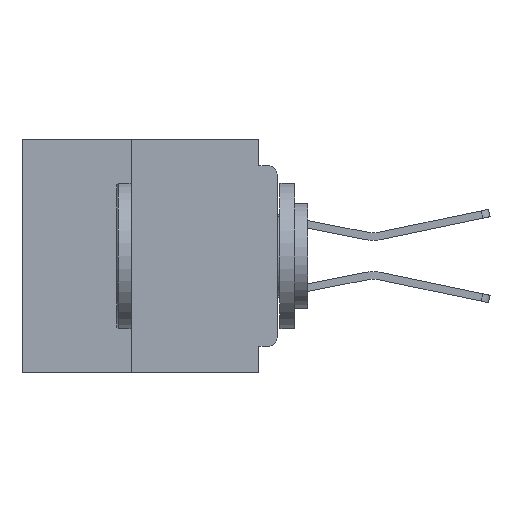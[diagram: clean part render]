
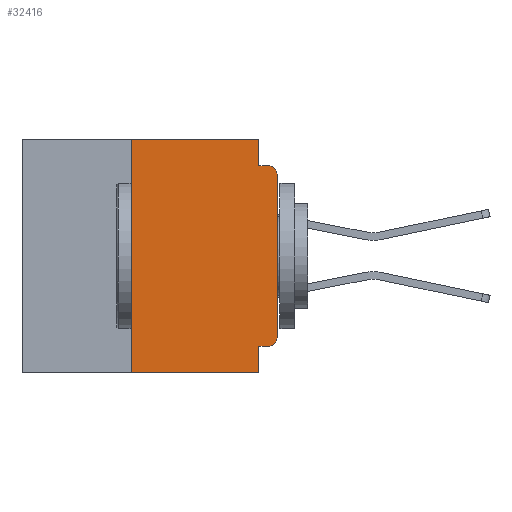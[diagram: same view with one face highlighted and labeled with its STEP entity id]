
A CAD part, left-side view. The second image highlights one B-rep face of the part: STEP entity #32416.
In plain terms, the highlighted planar face has unit normal (-1, 0, 0).
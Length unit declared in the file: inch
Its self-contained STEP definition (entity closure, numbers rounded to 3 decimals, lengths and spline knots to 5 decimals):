
#83 = DIRECTION ( 'NONE',  ( 0., 1., 0. ) ) ;
#743 = DIRECTION ( 'NONE',  ( 1., 0., 0. ) ) ;
#1963 = DIRECTION ( 'NONE',  ( 0., 0., 1. ) ) ;
#2668 = LINE ( 'NONE', #30437, #31247 ) ;
#2755 = CARTESIAN_POINT ( 'NONE',  ( 0., 0., -0.06 ) ) ;
#3160 = CARTESIAN_POINT ( 'NONE',  ( 0., 0., -0.34 ) ) ;
#3500 = VECTOR ( 'NONE', #25372, 39.37008 ) ;
#4322 = VERTEX_POINT ( 'NONE', #23032 ) ;
#4366 = ORIENTED_EDGE ( 'NONE', *, *, #6041, .T. ) ;
#4501 = VERTEX_POINT ( 'NONE', #12725 ) ;
#5192 = DIRECTION ( 'NONE',  ( 0., 0., -1. ) ) ;
#5506 = CIRCLE ( 'NONE', #24848, 0.015 ) ;
#5573 = AXIS2_PLACEMENT_3D ( 'NONE', #29106, #743, #20757 ) ;
#5625 = CARTESIAN_POINT ( 'NONE',  ( 0., 0.015, -0.34 ) ) ;
#5630 = VERTEX_POINT ( 'NONE', #25445 ) ;
#5817 = CARTESIAN_POINT ( 'NONE',  ( 0., 0., -0.045 ) ) ;
#6041 = EDGE_CURVE ( 'NONE', #14646, #21841, #5506, .T. ) ;
#6405 = VECTOR ( 'NONE', #10740, 39.37008 ) ;
#7563 = LINE ( 'NONE', #19468, #14278 ) ;
#8063 = ORIENTED_EDGE ( 'NONE', *, *, #14201, .F. ) ;
#8488 = DIRECTION ( 'NONE',  ( 0., 0., -1. ) ) ;
#8681 = ORIENTED_EDGE ( 'NONE', *, *, #33311, .F. ) ;
#8688 = DIRECTION ( 'NONE',  ( 0., -1., 0. ) ) ;
#9278 = EDGE_CURVE ( 'NONE', #18336, #19680, #32067, .T. ) ;
#9790 = ORIENTED_EDGE ( 'NONE', *, *, #28148, .T. ) ;
#10420 = CARTESIAN_POINT ( 'NONE',  ( 0., 0.015, -0.06 ) ) ;
#10566 = CARTESIAN_POINT ( 'NONE',  ( 0., 0.015, -0.045 ) ) ;
#10740 = DIRECTION ( 'NONE',  ( 0., -1., 0. ) ) ;
#10999 = LINE ( 'NONE', #26510, #32918 ) ;
#12725 = CARTESIAN_POINT ( 'NONE',  ( 0., 0.031, -0.355 ) ) ;
#13320 = DIRECTION ( 'NONE',  ( 0., 0., -1. ) ) ;
#13360 = LINE ( 'NONE', #16073, #27629 ) ;
#13457 = EDGE_CURVE ( 'NONE', #18336, #4501, #20926, .T. ) ;
#13464 = EDGE_CURVE ( 'NONE', #14717, #21841, #20031, .T. ) ;
#14201 = EDGE_CURVE ( 'NONE', #30999, #5630, #10999, .T. ) ;
#14278 = VECTOR ( 'NONE', #5192, 39.37008 ) ;
#14338 = CARTESIAN_POINT ( 'NONE',  ( 0., 0.25, -0.4 ) ) ;
#14646 = VERTEX_POINT ( 'NONE', #2755 ) ;
#14717 = VERTEX_POINT ( 'NONE', #31594 ) ;
#15000 = PLANE ( 'NONE',  #5573 ) ;
#16073 = CARTESIAN_POINT ( 'NONE',  ( 0., 0.031, -0.4 ) ) ;
#16551 = FACE_OUTER_BOUND ( 'NONE', #33145, .T. ) ;
#16702 = ORIENTED_EDGE ( 'NONE', *, *, #34059, .F. ) ;
#17923 = DIRECTION ( 'NONE',  ( 0., 0., 1. ) ) ;
#18336 = VERTEX_POINT ( 'NONE', #34581 ) ;
#19468 = CARTESIAN_POINT ( 'NONE',  ( 0., 0.031, 0. ) ) ;
#19680 = VERTEX_POINT ( 'NONE', #3160 ) ;
#20031 = LINE ( 'NONE', #5817, #34292 ) ;
#20757 = DIRECTION ( 'NONE',  ( 0., 0., -1. ) ) ;
#20926 = LINE ( 'NONE', #34291, #27590 ) ;
#21810 = DIRECTION ( 'NONE',  ( 0., 0., -1. ) ) ;
#21841 = VERTEX_POINT ( 'NONE', #10566 ) ;
#22518 = CARTESIAN_POINT ( 'NONE',  ( 0., 0.437, 0. ) ) ;
#23032 = CARTESIAN_POINT ( 'NONE',  ( 0., 0.031, 0. ) ) ;
#24848 = AXIS2_PLACEMENT_3D ( 'NONE', #10420, #30424, #13320 ) ;
#25372 = DIRECTION ( 'NONE',  ( 0., -1., 0. ) ) ;
#25445 = CARTESIAN_POINT ( 'NONE',  ( 0., 0.25, 0. ) ) ;
#25582 = EDGE_CURVE ( 'NONE', #4501, #34834, #13360, .T. ) ;
#25607 = DIRECTION ( 'NONE',  ( -1., 0., 0. ) ) ;
#26098 = ORIENTED_EDGE ( 'NONE', *, *, #13464, .F. ) ;
#26510 = CARTESIAN_POINT ( 'NONE',  ( 0., 0.25, -0.4 ) ) ;
#27590 = VECTOR ( 'NONE', #83, 39.37008 ) ;
#27629 = VECTOR ( 'NONE', #21810, 39.37008 ) ;
#28148 = EDGE_CURVE ( 'NONE', #30999, #34834, #36773, .T. ) ;
#29106 = CARTESIAN_POINT ( 'NONE',  ( 0., 0.437, 0. ) ) ;
#30424 = DIRECTION ( 'NONE',  ( -1., 0., 0. ) ) ;
#30437 = CARTESIAN_POINT ( 'NONE',  ( 0., 0., 0. ) ) ;
#30999 = VERTEX_POINT ( 'NONE', #14338 ) ;
#31014 = ORIENTED_EDGE ( 'NONE', *, *, #25582, .F. ) ;
#31247 = VECTOR ( 'NONE', #1963, 39.37008 ) ;
#31594 = CARTESIAN_POINT ( 'NONE',  ( 0., 0.031, -0.045 ) ) ;
#32067 = CIRCLE ( 'NONE', #32343, 0.015 ) ;
#32343 = AXIS2_PLACEMENT_3D ( 'NONE', #5625, #25607, #8488 ) ;
#32416 = ADVANCED_FACE ( 'NONE', ( #16551 ), #15000, .F. ) ;
#32918 = VECTOR ( 'NONE', #17923, 39.37008 ) ;
#33145 = EDGE_LOOP ( 'NONE', ( #35215, #4366, #26098, #8681, #16702, #8063, #9790, #31014, #33852, #34812 ) ) ;
#33246 = EDGE_CURVE ( 'NONE', #19680, #14646, #2668, .T. ) ;
#33311 = EDGE_CURVE ( 'NONE', #4322, #14717, #7563, .T. ) ;
#33612 = CARTESIAN_POINT ( 'NONE',  ( 0., 0.437, -0.4 ) ) ;
#33852 = ORIENTED_EDGE ( 'NONE', *, *, #13457, .F. ) ;
#33883 = LINE ( 'NONE', #22518, #3500 ) ;
#34059 = EDGE_CURVE ( 'NONE', #5630, #4322, #33883, .T. ) ;
#34291 = CARTESIAN_POINT ( 'NONE',  ( 0., 0., -0.355 ) ) ;
#34292 = VECTOR ( 'NONE', #8688, 39.37008 ) ;
#34581 = CARTESIAN_POINT ( 'NONE',  ( 0., 0.015, -0.355 ) ) ;
#34812 = ORIENTED_EDGE ( 'NONE', *, *, #9278, .T. ) ;
#34834 = VERTEX_POINT ( 'NONE', #36653 ) ;
#35215 = ORIENTED_EDGE ( 'NONE', *, *, #33246, .T. ) ;
#36653 = CARTESIAN_POINT ( 'NONE',  ( 0., 0.031, -0.4 ) ) ;
#36773 = LINE ( 'NONE', #33612, #6405 ) ;
